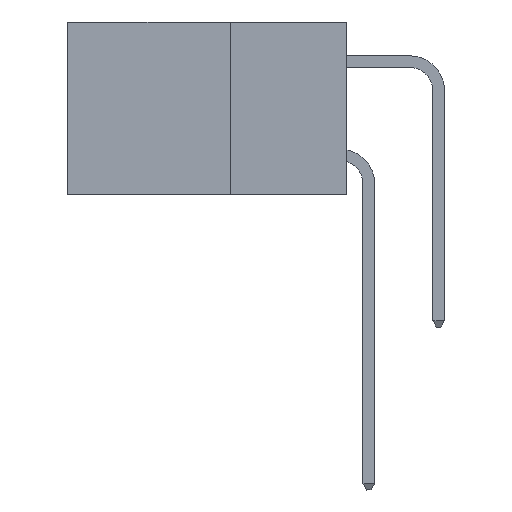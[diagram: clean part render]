
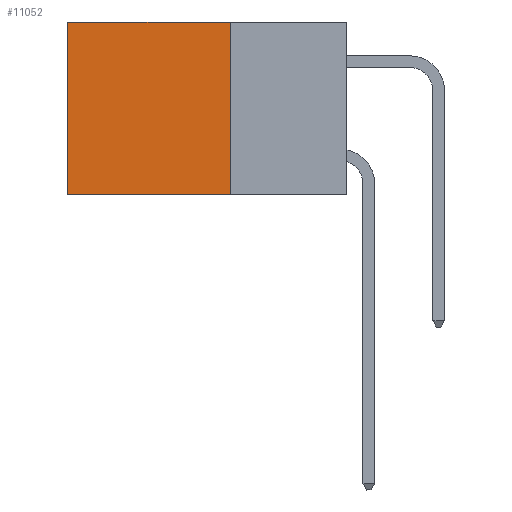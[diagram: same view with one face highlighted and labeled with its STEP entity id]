
A CAD part, left-side view. The second image highlights one B-rep face of the part: STEP entity #11052.
In plain terms, the highlighted planar face has unit normal (-1, 0, 0).
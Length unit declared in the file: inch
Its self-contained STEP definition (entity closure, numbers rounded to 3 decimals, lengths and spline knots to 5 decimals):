
#2410 = LINE ( 'NONE', #9082, #21234 ) ;
#2748 = DIRECTION ( 'NONE',  ( 0., 1., 0. ) ) ;
#3591 = CARTESIAN_POINT ( 'NONE',  ( 0.2875, 0.25, 0. ) ) ;
#4415 = CARTESIAN_POINT ( 'NONE',  ( 0.2875, 0.6, -0.37 ) ) ;
#5418 = DIRECTION ( 'NONE',  ( 0., 0., -1. ) ) ;
#5587 = CARTESIAN_POINT ( 'NONE',  ( 0.2875, 0.25, -0.37 ) ) ;
#9082 = CARTESIAN_POINT ( 'NONE',  ( 0.2875, 0.25, -0.37 ) ) ;
#10380 = CARTESIAN_POINT ( 'NONE',  ( 0.2875, 0.25, 0. ) ) ;
#11052 = ADVANCED_FACE ( 'NONE', ( #30830 ), #26429, .F. ) ;
#11576 = VECTOR ( 'NONE', #5418, 39.37008 ) ;
#11946 = CARTESIAN_POINT ( 'NONE',  ( 0.2875, 0.25, 0. ) ) ;
#12102 = EDGE_CURVE ( 'NONE', #36701, #36233, #23758, .T. ) ;
#13546 = DIRECTION ( 'NONE',  ( 0., 0., -1. ) ) ;
#13650 = DIRECTION ( 'NONE',  ( 0., 0., -1. ) ) ;
#13727 = ORIENTED_EDGE ( 'NONE', *, *, #12102, .T. ) ;
#14121 = ORIENTED_EDGE ( 'NONE', *, *, #25483, .T. ) ;
#14549 = ORIENTED_EDGE ( 'NONE', *, *, #21328, .F. ) ;
#16191 = VECTOR ( 'NONE', #13650, 39.37008 ) ;
#18436 = CARTESIAN_POINT ( 'NONE',  ( 0.2875, 0.6, 0. ) ) ;
#19976 = LINE ( 'NONE', #11946, #11576 ) ;
#20176 = LINE ( 'NONE', #23088, #16191 ) ;
#21234 = VECTOR ( 'NONE', #21542, 39.37008 ) ;
#21328 = EDGE_CURVE ( 'NONE', #36701, #36081, #19976, .T. ) ;
#21445 = AXIS2_PLACEMENT_3D ( 'NONE', #10380, #29378, #13546 ) ;
#21542 = DIRECTION ( 'NONE',  ( 0., 1., 0. ) ) ;
#23088 = CARTESIAN_POINT ( 'NONE',  ( 0.2875, 0.6, 0. ) ) ;
#23758 = LINE ( 'NONE', #3591, #26731 ) ;
#25483 = EDGE_CURVE ( 'NONE', #36233, #26056, #20176, .T. ) ;
#26056 = VERTEX_POINT ( 'NONE', #4415 ) ;
#26429 = PLANE ( 'NONE',  #21445 ) ;
#26731 = VECTOR ( 'NONE', #2748, 39.37008 ) ;
#27853 = CARTESIAN_POINT ( 'NONE',  ( 0.2875, 0.25, 0. ) ) ;
#29378 = DIRECTION ( 'NONE',  ( 1., 0., 0. ) ) ;
#30830 = FACE_OUTER_BOUND ( 'NONE', #32458, .T. ) ;
#31704 = EDGE_CURVE ( 'NONE', #36081, #26056, #2410, .T. ) ;
#32458 = EDGE_LOOP ( 'NONE', ( #14121, #40779, #14549, #13727 ) ) ;
#36081 = VERTEX_POINT ( 'NONE', #5587 ) ;
#36233 = VERTEX_POINT ( 'NONE', #18436 ) ;
#36701 = VERTEX_POINT ( 'NONE', #27853 ) ;
#40779 = ORIENTED_EDGE ( 'NONE', *, *, #31704, .F. ) ;
